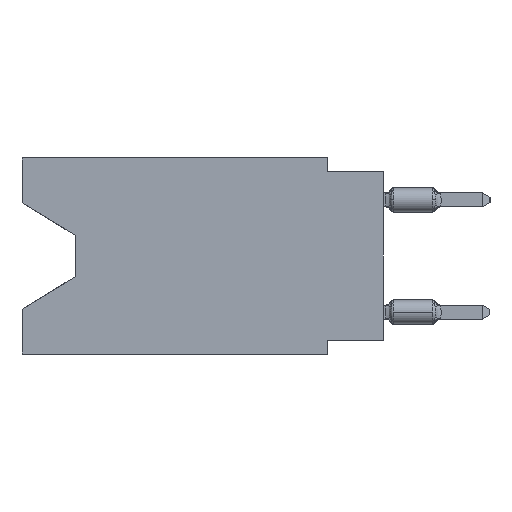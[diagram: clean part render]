
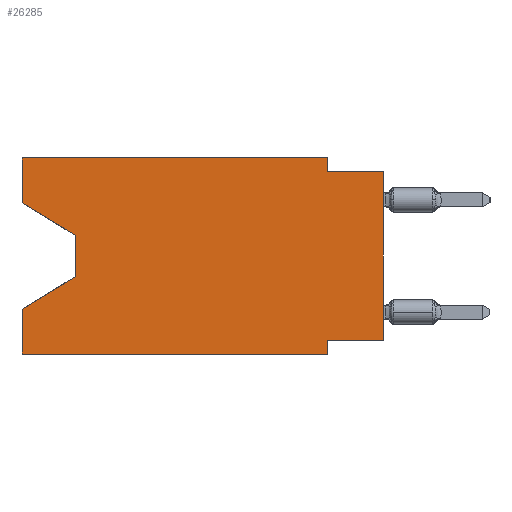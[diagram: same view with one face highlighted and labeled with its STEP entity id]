
A CAD part, left-side view. The second image highlights one B-rep face of the part: STEP entity #26285.
In plain terms, the highlighted planar face has unit normal (-1, 0, 0).
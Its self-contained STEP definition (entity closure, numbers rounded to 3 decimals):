
#170 = CARTESIAN_POINT ( 'NONE',  ( 0., 0., -0.635 ) ) ;
#466 = LINE ( 'NONE', #37806, #30538 ) ;
#584 = EDGE_CURVE ( 'NONE', #32051, #29470, #24934, .T. ) ;
#1571 = CARTESIAN_POINT ( 'NONE',  ( 0., 0., -0.635 ) ) ;
#1771 = EDGE_CURVE ( 'NONE', #7793, #2373, #30668, .T. ) ;
#1965 = VERTEX_POINT ( 'NONE', #14791 ) ;
#2058 = CARTESIAN_POINT ( 'NONE',  ( 0., 0., -8.255 ) ) ;
#2209 = EDGE_LOOP ( 'NONE', ( #25400, #40117, #10347, #36441, #19248, #28368, #14217, #3921, #31900, #22882, #35184, #2396 ) ) ;
#2329 = LINE ( 'NONE', #32996, #4034 ) ;
#2340 = LINE ( 'NONE', #30904, #29335 ) ;
#2373 = VERTEX_POINT ( 'NONE', #24032 ) ;
#2396 = ORIENTED_EDGE ( 'NONE', *, *, #9567, .F. ) ;
#2839 = VECTOR ( 'NONE', #17334, 1000. ) ;
#3005 = CARTESIAN_POINT ( 'NONE',  ( 0., 13.97, -5.385 ) ) ;
#3096 = PLANE ( 'NONE',  #26136 ) ;
#3504 = LINE ( 'NONE', #3700, #10568 ) ;
#3700 = CARTESIAN_POINT ( 'NONE',  ( 0., 16.383, -2.038 ) ) ;
#3822 = EDGE_CURVE ( 'NONE', #12489, #7793, #466, .T. ) ;
#3921 = ORIENTED_EDGE ( 'NONE', *, *, #16922, .T. ) ;
#4034 = VECTOR ( 'NONE', #24251, 1000. ) ;
#4238 = CARTESIAN_POINT ( 'NONE',  ( 0., 16.383, -8.89 ) ) ;
#4351 = CARTESIAN_POINT ( 'NONE',  ( 0., 16.383, 0. ) ) ;
#4941 = CARTESIAN_POINT ( 'NONE',  ( 0., 16.383, 0. ) ) ;
#6294 = DIRECTION ( 'NONE',  ( 0., 0.855, -0.519 ) ) ;
#7340 = DIRECTION ( 'NONE',  ( 0., -0.855, -0.519 ) ) ;
#7793 = VERTEX_POINT ( 'NONE', #3005 ) ;
#8385 = CARTESIAN_POINT ( 'NONE',  ( 0., 13.97, -3.505 ) ) ;
#8640 = CARTESIAN_POINT ( 'NONE',  ( 0., 2.54, -8.89 ) ) ;
#9567 = EDGE_CURVE ( 'NONE', #17806, #33985, #25890, .T. ) ;
#9603 = VECTOR ( 'NONE', #19224, 1000. ) ;
#10347 = ORIENTED_EDGE ( 'NONE', *, *, #1771, .T. ) ;
#10568 = VECTOR ( 'NONE', #7340, 1000. ) ;
#10628 = EDGE_CURVE ( 'NONE', #33000, #1965, #34082, .T. ) ;
#11304 = CARTESIAN_POINT ( 'NONE',  ( 0., 16.383, 0. ) ) ;
#11411 = VECTOR ( 'NONE', #34869, 1000. ) ;
#12427 = DIRECTION ( 'NONE',  ( 0., 0., 1. ) ) ;
#12489 = VERTEX_POINT ( 'NONE', #8385 ) ;
#14009 = EDGE_CURVE ( 'NONE', #22847, #34351, #36992, .T. ) ;
#14217 = ORIENTED_EDGE ( 'NONE', *, *, #10628, .F. ) ;
#14791 = CARTESIAN_POINT ( 'NONE',  ( 0., 2.54, -8.255 ) ) ;
#15479 = DIRECTION ( 'NONE',  ( 1., 0., 0. ) ) ;
#16922 = EDGE_CURVE ( 'NONE', #33000, #36093, #2340, .T. ) ;
#17081 = VECTOR ( 'NONE', #19994, 1000. ) ;
#17334 = DIRECTION ( 'NONE',  ( 0., 0., 1. ) ) ;
#17806 = VERTEX_POINT ( 'NONE', #24113 ) ;
#18525 = FACE_OUTER_BOUND ( 'NONE', #2209, .T. ) ;
#18722 = CARTESIAN_POINT ( 'NONE',  ( 0., 16.383, 0. ) ) ;
#19224 = DIRECTION ( 'NONE',  ( 0., -1., 0. ) ) ;
#19248 = ORIENTED_EDGE ( 'NONE', *, *, #584, .T. ) ;
#19994 = DIRECTION ( 'NONE',  ( 0., 0., 1. ) ) ;
#20171 = EDGE_CURVE ( 'NONE', #1965, #29470, #2329, .T. ) ;
#21583 = CARTESIAN_POINT ( 'NONE',  ( 0., 2.54, 0. ) ) ;
#22178 = EDGE_CURVE ( 'NONE', #33985, #22847, #31896, .T. ) ;
#22287 = CARTESIAN_POINT ( 'NONE',  ( 0., 16.383, -8.89 ) ) ;
#22847 = VERTEX_POINT ( 'NONE', #38721 ) ;
#22882 = ORIENTED_EDGE ( 'NONE', *, *, #14009, .F. ) ;
#24032 = CARTESIAN_POINT ( 'NONE',  ( 0., 16.383, -6.852 ) ) ;
#24113 = CARTESIAN_POINT ( 'NONE',  ( 0., 16.383, -2.038 ) ) ;
#24251 = DIRECTION ( 'NONE',  ( 0., 0., -1. ) ) ;
#24934 = LINE ( 'NONE', #22287, #9603 ) ;
#25400 = ORIENTED_EDGE ( 'NONE', *, *, #26424, .T. ) ;
#25636 = DIRECTION ( 'NONE',  ( 0., 0., -1. ) ) ;
#25890 = LINE ( 'NONE', #4351, #17081 ) ;
#26136 = AXIS2_PLACEMENT_3D ( 'NONE', #18722, #15479, #27253 ) ;
#26172 = EDGE_CURVE ( 'NONE', #32051, #2373, #32767, .T. ) ;
#26285 = ADVANCED_FACE ( 'NONE', ( #18525 ), #3096, .F. ) ;
#26424 = EDGE_CURVE ( 'NONE', #17806, #12489, #3504, .T. ) ;
#27253 = DIRECTION ( 'NONE',  ( 0., 0., -1. ) ) ;
#27443 = VECTOR ( 'NONE', #34347, 1000. ) ;
#28368 = ORIENTED_EDGE ( 'NONE', *, *, #20171, .F. ) ;
#28577 = LINE ( 'NONE', #170, #11411 ) ;
#28852 = DIRECTION ( 'NONE',  ( 0., -1., 0. ) ) ;
#29016 = VECTOR ( 'NONE', #28852, 1000. ) ;
#29335 = VECTOR ( 'NONE', #12427, 1000. ) ;
#29470 = VERTEX_POINT ( 'NONE', #8640 ) ;
#30538 = VECTOR ( 'NONE', #25636, 1000. ) ;
#30668 = LINE ( 'NONE', #36950, #31070 ) ;
#30904 = CARTESIAN_POINT ( 'NONE',  ( 0., 0., 0. ) ) ;
#31070 = VECTOR ( 'NONE', #6294, 1000. ) ;
#31896 = LINE ( 'NONE', #32100, #29016 ) ;
#31900 = ORIENTED_EDGE ( 'NONE', *, *, #35976, .F. ) ;
#32051 = VERTEX_POINT ( 'NONE', #4238 ) ;
#32100 = CARTESIAN_POINT ( 'NONE',  ( 0., 16.383, 0. ) ) ;
#32767 = LINE ( 'NONE', #4941, #2839 ) ;
#32996 = CARTESIAN_POINT ( 'NONE',  ( 0., 2.54, -8.89 ) ) ;
#33000 = VERTEX_POINT ( 'NONE', #2058 ) ;
#33480 = DIRECTION ( 'NONE',  ( 0., 1., 0. ) ) ;
#33875 = CARTESIAN_POINT ( 'NONE',  ( 0., 0., -8.255 ) ) ;
#33985 = VERTEX_POINT ( 'NONE', #11304 ) ;
#34082 = LINE ( 'NONE', #33875, #39842 ) ;
#34347 = DIRECTION ( 'NONE',  ( 0., 0., -1. ) ) ;
#34351 = VERTEX_POINT ( 'NONE', #39997 ) ;
#34869 = DIRECTION ( 'NONE',  ( 0., -1., 0. ) ) ;
#35184 = ORIENTED_EDGE ( 'NONE', *, *, #22178, .F. ) ;
#35976 = EDGE_CURVE ( 'NONE', #34351, #36093, #28577, .T. ) ;
#36093 = VERTEX_POINT ( 'NONE', #1571 ) ;
#36441 = ORIENTED_EDGE ( 'NONE', *, *, #26172, .F. ) ;
#36950 = CARTESIAN_POINT ( 'NONE',  ( 0., 13.97, -5.385 ) ) ;
#36992 = LINE ( 'NONE', #21583, #27443 ) ;
#37806 = CARTESIAN_POINT ( 'NONE',  ( 0., 13.97, -3.505 ) ) ;
#38721 = CARTESIAN_POINT ( 'NONE',  ( 0., 2.54, 0. ) ) ;
#39842 = VECTOR ( 'NONE', #33480, 1000. ) ;
#39997 = CARTESIAN_POINT ( 'NONE',  ( 0., 2.54, -0.635 ) ) ;
#40117 = ORIENTED_EDGE ( 'NONE', *, *, #3822, .T. ) ;
